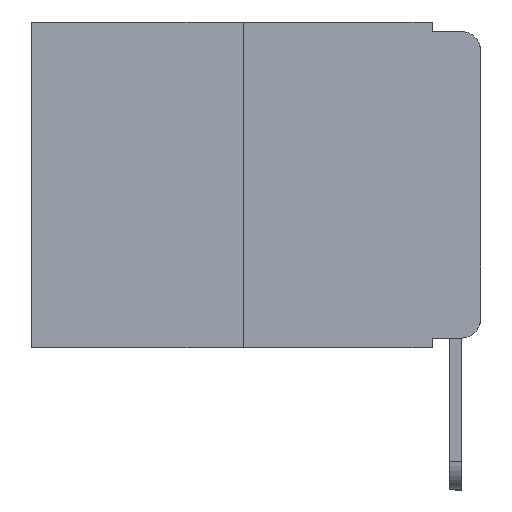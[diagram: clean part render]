
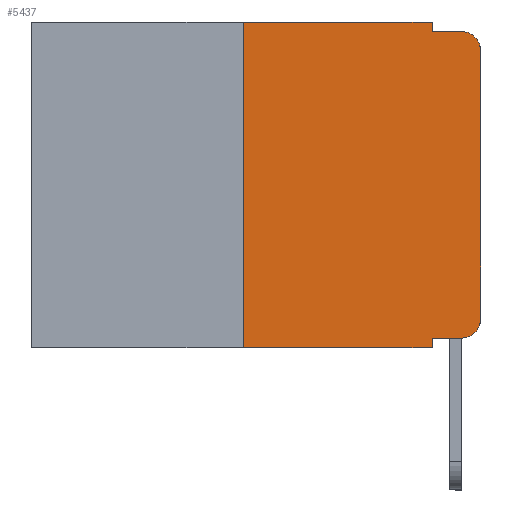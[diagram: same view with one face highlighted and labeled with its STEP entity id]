
A CAD part, left-side view. The second image highlights one B-rep face of the part: STEP entity #5437.
In plain terms, the highlighted planar face has unit normal (-1, 0, 0).
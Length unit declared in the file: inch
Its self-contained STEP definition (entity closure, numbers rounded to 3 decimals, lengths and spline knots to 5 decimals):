
#26 = EDGE_CURVE ( 'NONE', #8319, #5729, #18036, .T. ) ;
#392 = CARTESIAN_POINT ( 'NONE',  ( 0., 0.25, -0.343 ) ) ;
#844 = AXIS2_PLACEMENT_3D ( 'NONE', #4274, #4522, #19389 ) ;
#1887 = AXIS2_PLACEMENT_3D ( 'NONE', #10288, #10166, #23663 ) ;
#2027 = EDGE_CURVE ( 'NONE', #2312, #7724, #11798, .T. ) ;
#2060 = CIRCLE ( 'NONE', #8326, 0.02 ) ;
#2256 = CIRCLE ( 'NONE', #1887, 0.02 ) ;
#2312 = VERTEX_POINT ( 'NONE', #7396 ) ;
#2331 = CARTESIAN_POINT ( 'NONE',  ( 0., 0.051, -0.333 ) ) ;
#2518 = DIRECTION ( 'NONE',  ( 0., -1., 0. ) ) ;
#3280 = ORIENTED_EDGE ( 'NONE', *, *, #11679, .T. ) ;
#3689 = VERTEX_POINT ( 'NONE', #7401 ) ;
#4091 = DIRECTION ( 'NONE',  ( -1., 0., 0. ) ) ;
#4274 = CARTESIAN_POINT ( 'NONE',  ( 0., 0.473, 0. ) ) ;
#4522 = DIRECTION ( 'NONE',  ( 1., 0., 0. ) ) ;
#4838 = CARTESIAN_POINT ( 'NONE',  ( 0., 0.02, -0.333 ) ) ;
#5437 = ADVANCED_FACE ( 'NONE', ( #23068 ), #7737, .F. ) ;
#5729 = VERTEX_POINT ( 'NONE', #24040 ) ;
#5892 = CARTESIAN_POINT ( 'NONE',  ( 0., 0., 0. ) ) ;
#5927 = VECTOR ( 'NONE', #8149, 39.37008 ) ;
#6155 = CARTESIAN_POINT ( 'NONE',  ( 0., 0.25, 0. ) ) ;
#7032 = DIRECTION ( 'NONE',  ( 0., -1., 0. ) ) ;
#7141 = VECTOR ( 'NONE', #8894, 39.37008 ) ;
#7301 = ORIENTED_EDGE ( 'NONE', *, *, #7845, .T. ) ;
#7396 = CARTESIAN_POINT ( 'NONE',  ( 0., 0.25, 0. ) ) ;
#7401 = CARTESIAN_POINT ( 'NONE',  ( 0., 0.02, -0.01 ) ) ;
#7561 = ORIENTED_EDGE ( 'NONE', *, *, #13395, .T. ) ;
#7724 = VERTEX_POINT ( 'NONE', #15555 ) ;
#7737 = PLANE ( 'NONE',  #844 ) ;
#7828 = CARTESIAN_POINT ( 'NONE',  ( 0., 0., -0.313 ) ) ;
#7845 = EDGE_CURVE ( 'NONE', #19226, #5729, #18015, .T. ) ;
#8149 = DIRECTION ( 'NONE',  ( 0., 0., 1. ) ) ;
#8319 = VERTEX_POINT ( 'NONE', #14621 ) ;
#8326 = AXIS2_PLACEMENT_3D ( 'NONE', #15388, #4091, #19439 ) ;
#8848 = VECTOR ( 'NONE', #19875, 39.37008 ) ;
#8894 = DIRECTION ( 'NONE',  ( 0., 0., -1. ) ) ;
#9791 = EDGE_CURVE ( 'NONE', #19226, #2312, #20923, .T. ) ;
#9796 = DIRECTION ( 'NONE',  ( 0., -1., 0. ) ) ;
#10166 = DIRECTION ( 'NONE',  ( -1., 0., 0. ) ) ;
#10288 = CARTESIAN_POINT ( 'NONE',  ( 0., 0.02, -0.03 ) ) ;
#11337 = EDGE_LOOP ( 'NONE', ( #7561, #19441, #12192, #18803, #11362, #23042, #7301, #17766, #21349, #3280 ) ) ;
#11362 = ORIENTED_EDGE ( 'NONE', *, *, #2027, .F. ) ;
#11679 = EDGE_CURVE ( 'NONE', #19833, #24133, #2060, .T. ) ;
#11795 = EDGE_CURVE ( 'NONE', #7724, #15200, #14255, .T. ) ;
#11798 = LINE ( 'NONE', #19433, #14548 ) ;
#12192 = ORIENTED_EDGE ( 'NONE', *, *, #15745, .F. ) ;
#13053 = VECTOR ( 'NONE', #7032, 39.37008 ) ;
#13395 = EDGE_CURVE ( 'NONE', #24133, #19360, #22737, .T. ) ;
#13801 = CARTESIAN_POINT ( 'NONE',  ( 0., 0.051, -0.01 ) ) ;
#13821 = CARTESIAN_POINT ( 'NONE',  ( 0., 0., -0.03 ) ) ;
#13991 = CARTESIAN_POINT ( 'NONE',  ( 0., 0.051, 0. ) ) ;
#14175 = CARTESIAN_POINT ( 'NONE',  ( 0., 0.473, -0.343 ) ) ;
#14255 = LINE ( 'NONE', #13991, #7141 ) ;
#14548 = VECTOR ( 'NONE', #2518, 39.37008 ) ;
#14621 = CARTESIAN_POINT ( 'NONE',  ( 0., 0.051, -0.333 ) ) ;
#15200 = VERTEX_POINT ( 'NONE', #13801 ) ;
#15388 = CARTESIAN_POINT ( 'NONE',  ( 0., 0.02, -0.313 ) ) ;
#15555 = CARTESIAN_POINT ( 'NONE',  ( 0., 0.051, 0. ) ) ;
#15745 = EDGE_CURVE ( 'NONE', #15200, #3689, #18220, .T. ) ;
#16174 = DIRECTION ( 'NONE',  ( 0., -1., 0. ) ) ;
#17766 = ORIENTED_EDGE ( 'NONE', *, *, #26, .F. ) ;
#17778 = VECTOR ( 'NONE', #16174, 39.37008 ) ;
#18000 = VECTOR ( 'NONE', #9796, 39.37008 ) ;
#18015 = LINE ( 'NONE', #14175, #17778 ) ;
#18036 = LINE ( 'NONE', #23911, #8848 ) ;
#18220 = LINE ( 'NONE', #23851, #13053 ) ;
#18803 = ORIENTED_EDGE ( 'NONE', *, *, #11795, .F. ) ;
#19226 = VERTEX_POINT ( 'NONE', #392 ) ;
#19360 = VERTEX_POINT ( 'NONE', #13821 ) ;
#19369 = EDGE_CURVE ( 'NONE', #19360, #3689, #2256, .T. ) ;
#19389 = DIRECTION ( 'NONE',  ( 0., 0., -1. ) ) ;
#19433 = CARTESIAN_POINT ( 'NONE',  ( 0., 0.473, 0. ) ) ;
#19439 = DIRECTION ( 'NONE',  ( 0., 0., -1. ) ) ;
#19441 = ORIENTED_EDGE ( 'NONE', *, *, #19369, .T. ) ;
#19833 = VERTEX_POINT ( 'NONE', #4838 ) ;
#19875 = DIRECTION ( 'NONE',  ( 0., 0., -1. ) ) ;
#20907 = DIRECTION ( 'NONE',  ( 0., 0., 1. ) ) ;
#20923 = LINE ( 'NONE', #6155, #5927 ) ;
#20946 = VECTOR ( 'NONE', #20907, 39.37008 ) ;
#21114 = LINE ( 'NONE', #2331, #18000 ) ;
#21349 = ORIENTED_EDGE ( 'NONE', *, *, #22449, .T. ) ;
#22449 = EDGE_CURVE ( 'NONE', #8319, #19833, #21114, .T. ) ;
#22737 = LINE ( 'NONE', #5892, #20946 ) ;
#23042 = ORIENTED_EDGE ( 'NONE', *, *, #9791, .F. ) ;
#23068 = FACE_OUTER_BOUND ( 'NONE', #11337, .T. ) ;
#23663 = DIRECTION ( 'NONE',  ( 0., 0., -1. ) ) ;
#23851 = CARTESIAN_POINT ( 'NONE',  ( 0., 0.051, -0.01 ) ) ;
#23911 = CARTESIAN_POINT ( 'NONE',  ( 0., 0.051, 0. ) ) ;
#24040 = CARTESIAN_POINT ( 'NONE',  ( 0., 0.051, -0.343 ) ) ;
#24133 = VERTEX_POINT ( 'NONE', #7828 ) ;
